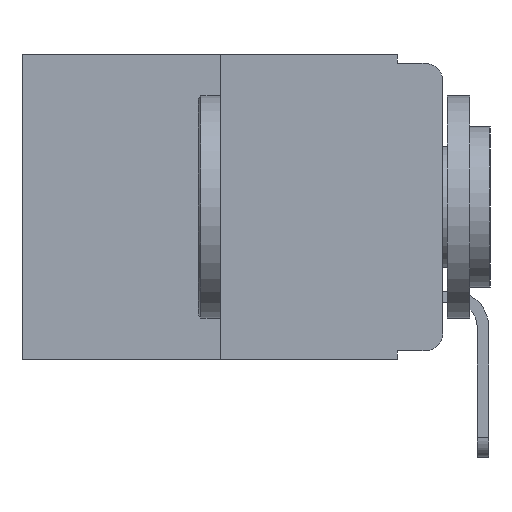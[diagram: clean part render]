
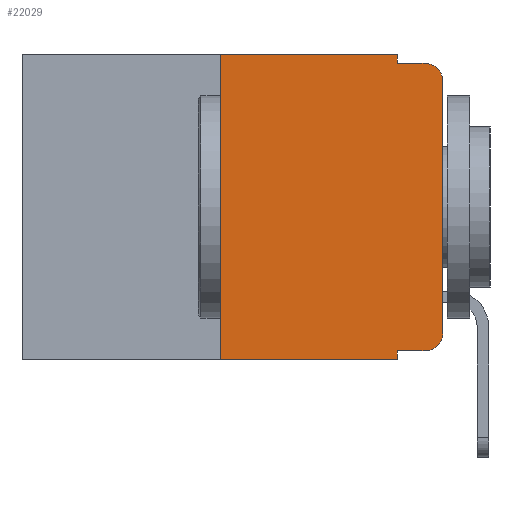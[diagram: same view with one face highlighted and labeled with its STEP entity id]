
A CAD part, left-side view. The second image highlights one B-rep face of the part: STEP entity #22029.
In plain terms, the highlighted planar face has unit normal (-1, 0, 0).
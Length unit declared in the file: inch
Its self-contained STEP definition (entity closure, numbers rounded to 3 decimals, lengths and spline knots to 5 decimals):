
#69 = DIRECTION ( 'NONE',  ( 0., -1., 0. ) ) ;
#1465 = CIRCLE ( 'NONE', #22958, 0.02 ) ;
#1736 = EDGE_CURVE ( 'NONE', #17668, #17275, #7293, .T. ) ;
#2407 = ORIENTED_EDGE ( 'NONE', *, *, #24102, .T. ) ;
#3451 = ORIENTED_EDGE ( 'NONE', *, *, #13368, .F. ) ;
#3569 = CARTESIAN_POINT ( 'NONE',  ( 0., 0.473, 0. ) ) ;
#4643 = EDGE_CURVE ( 'NONE', #17275, #7198, #1465, .T. ) ;
#4682 = VERTEX_POINT ( 'NONE', #15625 ) ;
#4912 = VERTEX_POINT ( 'NONE', #17188 ) ;
#5090 = LINE ( 'NONE', #7930, #21233 ) ;
#5364 = VERTEX_POINT ( 'NONE', #24125 ) ;
#5723 = CARTESIAN_POINT ( 'NONE',  ( 0., 0., -0.03 ) ) ;
#5980 = AXIS2_PLACEMENT_3D ( 'NONE', #13889, #20039, #7409 ) ;
#6464 = LINE ( 'NONE', #23168, #11660 ) ;
#7090 = VECTOR ( 'NONE', #11820, 39.37008 ) ;
#7198 = VERTEX_POINT ( 'NONE', #17580 ) ;
#7293 = LINE ( 'NONE', #17931, #12470 ) ;
#7409 = DIRECTION ( 'NONE',  ( 0., 0., -1. ) ) ;
#7472 = FACE_OUTER_BOUND ( 'NONE', #10831, .T. ) ;
#7514 = EDGE_CURVE ( 'NONE', #21168, #7198, #22688, .T. ) ;
#7680 = ORIENTED_EDGE ( 'NONE', *, *, #23774, .F. ) ;
#7795 = ORIENTED_EDGE ( 'NONE', *, *, #1736, .T. ) ;
#7913 = DIRECTION ( 'NONE',  ( 0., -1., 0. ) ) ;
#7930 = CARTESIAN_POINT ( 'NONE',  ( 0., 0.473, -0.343 ) ) ;
#8076 = ORIENTED_EDGE ( 'NONE', *, *, #4643, .T. ) ;
#8892 = LINE ( 'NONE', #10229, #15299 ) ;
#9149 = CARTESIAN_POINT ( 'NONE',  ( 0., 0.051, -0.01 ) ) ;
#9590 = PLANE ( 'NONE',  #5980 ) ;
#9932 = ORIENTED_EDGE ( 'NONE', *, *, #21556, .F. ) ;
#10102 = ORIENTED_EDGE ( 'NONE', *, *, #7514, .F. ) ;
#10229 = CARTESIAN_POINT ( 'NONE',  ( 0., 0.051, 0. ) ) ;
#10831 = EDGE_LOOP ( 'NONE', ( #7795, #8076, #10102, #3451, #7680, #20437, #24644, #9932, #2407, #23358 ) ) ;
#10887 = VECTOR ( 'NONE', #7913, 39.37008 ) ;
#11489 = CARTESIAN_POINT ( 'NONE',  ( 0., 0., -0.313 ) ) ;
#11660 = VECTOR ( 'NONE', #13134, 39.37008 ) ;
#11820 = DIRECTION ( 'NONE',  ( 0., 0., -1. ) ) ;
#12346 = DIRECTION ( 'NONE',  ( 0., 0., -1. ) ) ;
#12470 = VECTOR ( 'NONE', #17589, 39.37008 ) ;
#12939 = LINE ( 'NONE', #21979, #7090 ) ;
#12946 = CARTESIAN_POINT ( 'NONE',  ( 0., 0.02, -0.313 ) ) ;
#13134 = DIRECTION ( 'NONE',  ( 0., 0., 1. ) ) ;
#13349 = DIRECTION ( 'NONE',  ( 0., -1., 0. ) ) ;
#13368 = EDGE_CURVE ( 'NONE', #15905, #21168, #12939, .T. ) ;
#13419 = EDGE_CURVE ( 'NONE', #4682, #5364, #5090, .T. ) ;
#13538 = CARTESIAN_POINT ( 'NONE',  ( 0., 0.051, -0.333 ) ) ;
#13889 = CARTESIAN_POINT ( 'NONE',  ( 0., 0.473, 0. ) ) ;
#15058 = DIRECTION ( 'NONE',  ( 0., 0., -1. ) ) ;
#15299 = VECTOR ( 'NONE', #12346, 39.37008 ) ;
#15513 = VECTOR ( 'NONE', #69, 39.37008 ) ;
#15596 = DIRECTION ( 'NONE',  ( 0., 0., -1. ) ) ;
#15600 = DIRECTION ( 'NONE',  ( -1., 0., 0. ) ) ;
#15625 = CARTESIAN_POINT ( 'NONE',  ( 0., 0.25, -0.343 ) ) ;
#15905 = VERTEX_POINT ( 'NONE', #16634 ) ;
#16043 = CIRCLE ( 'NONE', #25997, 0.02 ) ;
#16332 = CARTESIAN_POINT ( 'NONE',  ( 0., 0.02, -0.03 ) ) ;
#16467 = LINE ( 'NONE', #3569, #10887 ) ;
#16634 = CARTESIAN_POINT ( 'NONE',  ( 0., 0.051, 0. ) ) ;
#16802 = VECTOR ( 'NONE', #13349, 39.37008 ) ;
#17188 = CARTESIAN_POINT ( 'NONE',  ( 0., 0.02, -0.333 ) ) ;
#17275 = VERTEX_POINT ( 'NONE', #5723 ) ;
#17547 = EDGE_CURVE ( 'NONE', #4682, #22632, #6464, .T. ) ;
#17580 = CARTESIAN_POINT ( 'NONE',  ( 0., 0.02, -0.01 ) ) ;
#17589 = DIRECTION ( 'NONE',  ( 0., 0., 1. ) ) ;
#17668 = VERTEX_POINT ( 'NONE', #11489 ) ;
#17931 = CARTESIAN_POINT ( 'NONE',  ( 0., 0., 0. ) ) ;
#19250 = CARTESIAN_POINT ( 'NONE',  ( 0., 0.051, -0.333 ) ) ;
#19921 = CARTESIAN_POINT ( 'NONE',  ( 0., 0.25, 0. ) ) ;
#20039 = DIRECTION ( 'NONE',  ( 1., 0., 0. ) ) ;
#20437 = ORIENTED_EDGE ( 'NONE', *, *, #17547, .F. ) ;
#21168 = VERTEX_POINT ( 'NONE', #21572 ) ;
#21233 = VECTOR ( 'NONE', #22569, 39.37008 ) ;
#21502 = LINE ( 'NONE', #19250, #15513 ) ;
#21556 = EDGE_CURVE ( 'NONE', #23612, #5364, #8892, .T. ) ;
#21572 = CARTESIAN_POINT ( 'NONE',  ( 0., 0.051, -0.01 ) ) ;
#21979 = CARTESIAN_POINT ( 'NONE',  ( 0., 0.051, 0. ) ) ;
#22029 = ADVANCED_FACE ( 'NONE', ( #7472 ), #9590, .F. ) ;
#22569 = DIRECTION ( 'NONE',  ( 0., -1., 0. ) ) ;
#22632 = VERTEX_POINT ( 'NONE', #19921 ) ;
#22688 = LINE ( 'NONE', #9149, #16802 ) ;
#22958 = AXIS2_PLACEMENT_3D ( 'NONE', #16332, #15600, #15596 ) ;
#23168 = CARTESIAN_POINT ( 'NONE',  ( 0., 0.25, 0. ) ) ;
#23358 = ORIENTED_EDGE ( 'NONE', *, *, #26662, .T. ) ;
#23612 = VERTEX_POINT ( 'NONE', #13538 ) ;
#23774 = EDGE_CURVE ( 'NONE', #22632, #15905, #16467, .T. ) ;
#24102 = EDGE_CURVE ( 'NONE', #23612, #4912, #21502, .T. ) ;
#24125 = CARTESIAN_POINT ( 'NONE',  ( 0., 0.051, -0.343 ) ) ;
#24644 = ORIENTED_EDGE ( 'NONE', *, *, #13419, .T. ) ;
#25997 = AXIS2_PLACEMENT_3D ( 'NONE', #12946, #26828, #15058 ) ;
#26662 = EDGE_CURVE ( 'NONE', #4912, #17668, #16043, .T. ) ;
#26828 = DIRECTION ( 'NONE',  ( -1., 0., 0. ) ) ;
